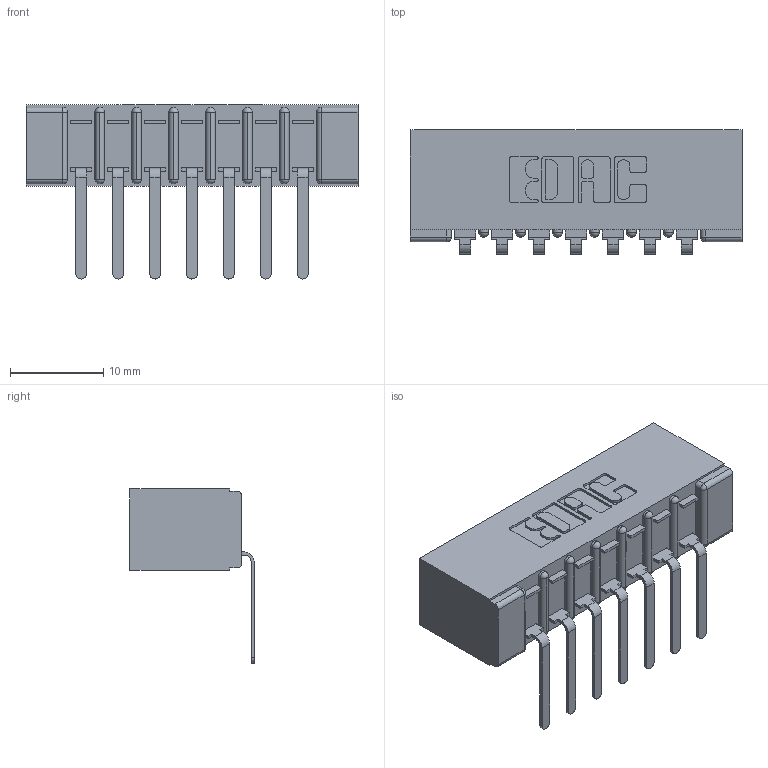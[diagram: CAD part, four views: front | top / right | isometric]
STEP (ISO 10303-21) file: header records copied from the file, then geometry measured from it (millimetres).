
FILE_DESCRIPTION (( 'STEP AP203' ), '1' );
FILE_NAME ('357-007-457-101.STEP', '2020-09-30T02:42:32', ( '' ), ( '' ), 'SwSTEP 2.0', 'SolidWorks 2020', '' );
FILE_SCHEMA (( 'CONFIG_CONTROL_DESIGN' ));
Length unit declared in the file: inch
Products named in the file (3): 307-290-002_557; 357-007-457-101; 307 Part_No Mounting Lugs
Assembly tree (8 placements, depth 2):
  357-007-457-101
    307 Part_No Mounting Lugs
    307-290-002_557  x7
Bounding box: 35.61 x 13.32 x 18.67 mm (x, y, z)
Volume: 2604.3 mm3; surface area: 4525.4 mm2
Topology: 8 solids, 8 shells, 664 faces, 2007 edges, 1314 vertices
Faces by surface type: plane 395, cylinder 253, sphere 16
Entity records: 10892 total; most frequent: CARTESIAN_POINT 1832, ORIENTED_EDGE 1822, DIRECTION 1795, EDGE_CURVE 911, LINE 681, VECTOR 681, VERTEX_POINT 594, AXIS2_PLACEMENT_3D 557
